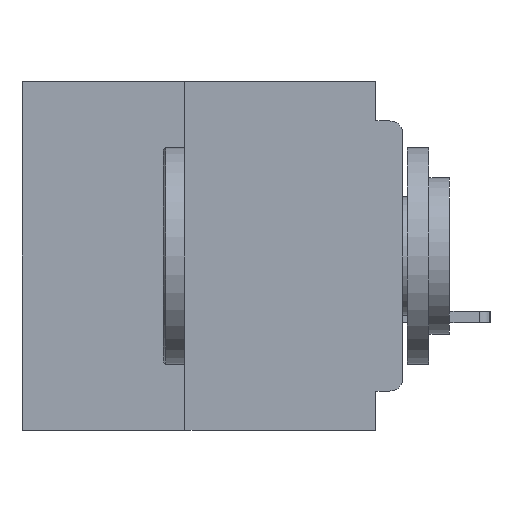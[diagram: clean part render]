
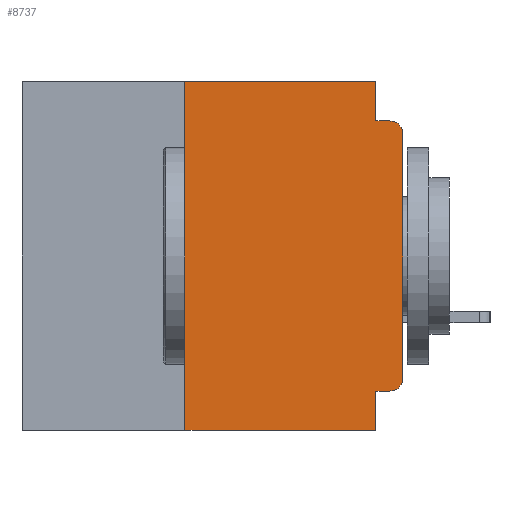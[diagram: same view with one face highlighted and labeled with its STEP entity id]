
A CAD part, left-side view. The second image highlights one B-rep face of the part: STEP entity #8737.
In plain terms, the highlighted planar face has unit normal (-1, 0, 0).
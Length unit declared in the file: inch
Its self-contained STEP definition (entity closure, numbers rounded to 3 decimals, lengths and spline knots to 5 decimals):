
#436 = ORIENTED_EDGE ( 'NONE', *, *, #12094, .F. ) ;
#631 = EDGE_CURVE ( 'NONE', #2610, #14303, #45735, .T. ) ;
#1434 = CARTESIAN_POINT ( 'NONE',  ( 0., 0., -0.355 ) ) ;
#1596 = EDGE_LOOP ( 'NONE', ( #31391, #39499, #3663, #42045, #47538, #37765, #20688, #436, #37323, #46347 ) ) ;
#2386 = VERTEX_POINT ( 'NONE', #46989 ) ;
#2610 = VERTEX_POINT ( 'NONE', #33787 ) ;
#3663 = ORIENTED_EDGE ( 'NONE', *, *, #18004, .F. ) ;
#5031 = FACE_OUTER_BOUND ( 'NONE', #1596, .T. ) ;
#5813 = VECTOR ( 'NONE', #15185, 39.37008 ) ;
#6369 = CARTESIAN_POINT ( 'NONE',  ( 0., 0.25, 0. ) ) ;
#7384 = DIRECTION ( 'NONE',  ( 0., -1., 0. ) ) ;
#7478 = LINE ( 'NONE', #22915, #27923 ) ;
#8567 = CARTESIAN_POINT ( 'NONE',  ( 0., 0.25, -0.4 ) ) ;
#8737 = ADVANCED_FACE ( 'NONE', ( #5031 ), #11529, .F. ) ;
#11529 = PLANE ( 'NONE',  #35709 ) ;
#12094 = EDGE_CURVE ( 'NONE', #28783, #14303, #16083, .T. ) ;
#12524 = DIRECTION ( 'NONE',  ( 0., 0., 1. ) ) ;
#13505 = LINE ( 'NONE', #1434, #31076 ) ;
#13966 = DIRECTION ( 'NONE',  ( 0., -1., 0. ) ) ;
#14303 = VERTEX_POINT ( 'NONE', #34934 ) ;
#14728 = VERTEX_POINT ( 'NONE', #19736 ) ;
#15185 = DIRECTION ( 'NONE',  ( 0., 0., -1. ) ) ;
#15663 = EDGE_CURVE ( 'NONE', #41271, #14728, #16415, .T. ) ;
#16083 = LINE ( 'NONE', #45139, #5813 ) ;
#16415 = CIRCLE ( 'NONE', #24456, 0.015 ) ;
#17299 = LINE ( 'NONE', #55189, #48698 ) ;
#18001 = CARTESIAN_POINT ( 'NONE',  ( 0., 0.437, -0.4 ) ) ;
#18004 = EDGE_CURVE ( 'NONE', #46350, #14728, #7478, .T. ) ;
#18145 = DIRECTION ( 'NONE',  ( -1., 0., 0. ) ) ;
#18531 = CARTESIAN_POINT ( 'NONE',  ( 0., 0.031, -0.045 ) ) ;
#19369 = VERTEX_POINT ( 'NONE', #6369 ) ;
#19736 = CARTESIAN_POINT ( 'NONE',  ( 0., 0.015, -0.045 ) ) ;
#20543 = LINE ( 'NONE', #8567, #49216 ) ;
#20688 = ORIENTED_EDGE ( 'NONE', *, *, #631, .T. ) ;
#22915 = CARTESIAN_POINT ( 'NONE',  ( 0., 0., -0.045 ) ) ;
#23226 = DIRECTION ( 'NONE',  ( 0., 0., -1. ) ) ;
#23229 = DIRECTION ( 'NONE',  ( 0., 1., 0. ) ) ;
#23711 = CARTESIAN_POINT ( 'NONE',  ( 0., 0.015, -0.34 ) ) ;
#24396 = VECTOR ( 'NONE', #13966, 39.37008 ) ;
#24456 = AXIS2_PLACEMENT_3D ( 'NONE', #43757, #18145, #47973 ) ;
#24687 = DIRECTION ( 'NONE',  ( 0., 0., -1. ) ) ;
#27923 = VECTOR ( 'NONE', #31540, 39.37008 ) ;
#28093 = DIRECTION ( 'NONE',  ( 0., 0., -1. ) ) ;
#28783 = VERTEX_POINT ( 'NONE', #39611 ) ;
#29487 = VERTEX_POINT ( 'NONE', #43350 ) ;
#31076 = VECTOR ( 'NONE', #23229, 39.37008 ) ;
#31391 = ORIENTED_EDGE ( 'NONE', *, *, #53961, .T. ) ;
#31540 = DIRECTION ( 'NONE',  ( 0., -1., 0. ) ) ;
#33129 = CARTESIAN_POINT ( 'NONE',  ( 0., 0.437, 0. ) ) ;
#33352 = CARTESIAN_POINT ( 'NONE',  ( 0., 0.437, 0. ) ) ;
#33787 = CARTESIAN_POINT ( 'NONE',  ( 0., 0.25, -0.4 ) ) ;
#34934 = CARTESIAN_POINT ( 'NONE',  ( 0., 0.031, -0.4 ) ) ;
#35709 = AXIS2_PLACEMENT_3D ( 'NONE', #33129, #50173, #24687 ) ;
#36154 = VECTOR ( 'NONE', #7384, 39.37008 ) ;
#37323 = ORIENTED_EDGE ( 'NONE', *, *, #44972, .F. ) ;
#37765 = ORIENTED_EDGE ( 'NONE', *, *, #42519, .F. ) ;
#39499 = ORIENTED_EDGE ( 'NONE', *, *, #15663, .T. ) ;
#39611 = CARTESIAN_POINT ( 'NONE',  ( 0., 0.031, -0.355 ) ) ;
#40355 = CIRCLE ( 'NONE', #40637, 0.015 ) ;
#40637 = AXIS2_PLACEMENT_3D ( 'NONE', #23711, #53472, #28093 ) ;
#41121 = EDGE_CURVE ( 'NONE', #19369, #50731, #48724, .T. ) ;
#41271 = VERTEX_POINT ( 'NONE', #43145 ) ;
#42045 = ORIENTED_EDGE ( 'NONE', *, *, #42759, .F. ) ;
#42519 = EDGE_CURVE ( 'NONE', #2610, #19369, #20543, .T. ) ;
#42759 = EDGE_CURVE ( 'NONE', #50731, #46350, #50605, .T. ) ;
#43009 = DIRECTION ( 'NONE',  ( 0., 0., 1. ) ) ;
#43145 = CARTESIAN_POINT ( 'NONE',  ( 0., 0., -0.06 ) ) ;
#43350 = CARTESIAN_POINT ( 'NONE',  ( 0., 0., -0.34 ) ) ;
#43757 = CARTESIAN_POINT ( 'NONE',  ( 0., 0.015, -0.06 ) ) ;
#44972 = EDGE_CURVE ( 'NONE', #2386, #28783, #13505, .T. ) ;
#45065 = CARTESIAN_POINT ( 'NONE',  ( 0., 0.031, 0. ) ) ;
#45139 = CARTESIAN_POINT ( 'NONE',  ( 0., 0.031, -0.4 ) ) ;
#45697 = EDGE_CURVE ( 'NONE', #2386, #29487, #40355, .T. ) ;
#45735 = LINE ( 'NONE', #18001, #24396 ) ;
#46347 = ORIENTED_EDGE ( 'NONE', *, *, #45697, .T. ) ;
#46350 = VERTEX_POINT ( 'NONE', #18531 ) ;
#46989 = CARTESIAN_POINT ( 'NONE',  ( 0., 0.015, -0.355 ) ) ;
#47538 = ORIENTED_EDGE ( 'NONE', *, *, #41121, .F. ) ;
#47931 = VECTOR ( 'NONE', #23226, 39.37008 ) ;
#47973 = DIRECTION ( 'NONE',  ( 0., 0., -1. ) ) ;
#48698 = VECTOR ( 'NONE', #12524, 39.37008 ) ;
#48724 = LINE ( 'NONE', #33352, #36154 ) ;
#49216 = VECTOR ( 'NONE', #43009, 39.37008 ) ;
#50173 = DIRECTION ( 'NONE',  ( 1., 0., 0. ) ) ;
#50605 = LINE ( 'NONE', #52983, #47931 ) ;
#50731 = VERTEX_POINT ( 'NONE', #45065 ) ;
#52983 = CARTESIAN_POINT ( 'NONE',  ( 0., 0.031, 0. ) ) ;
#53472 = DIRECTION ( 'NONE',  ( -1., 0., 0. ) ) ;
#53961 = EDGE_CURVE ( 'NONE', #29487, #41271, #17299, .T. ) ;
#55189 = CARTESIAN_POINT ( 'NONE',  ( 0., 0., 0. ) ) ;
